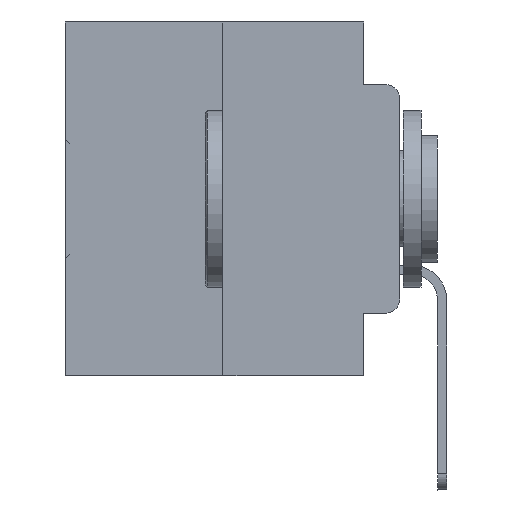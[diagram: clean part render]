
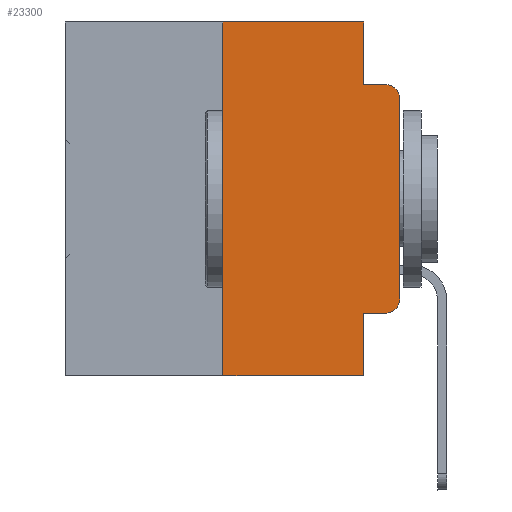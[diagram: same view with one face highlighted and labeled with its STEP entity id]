
A CAD part, left-side view. The second image highlights one B-rep face of the part: STEP entity #23300.
In plain terms, the highlighted planar face has unit normal (-1, 0, 0).
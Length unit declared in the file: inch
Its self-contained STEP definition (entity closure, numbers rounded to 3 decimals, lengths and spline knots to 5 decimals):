
#1575 = VERTEX_POINT ( 'NONE', #24179 ) ;
#1589 = EDGE_CURVE ( 'NONE', #19500, #1575, #29498, .T. ) ;
#2056 = CARTESIAN_POINT ( 'NONE',  ( 0., 0.473, 0. ) ) ;
#2067 = DIRECTION ( 'NONE',  ( 0., 0., 1. ) ) ;
#2554 = LINE ( 'NONE', #5208, #8796 ) ;
#2661 = CIRCLE ( 'NONE', #12740, 0.02 ) ;
#3149 = EDGE_CURVE ( 'NONE', #9847, #30426, #2661, .T. ) ;
#3550 = CARTESIAN_POINT ( 'NONE',  ( 0., 0.051, 0. ) ) ;
#4041 = CIRCLE ( 'NONE', #31563, 0.02 ) ;
#4110 = DIRECTION ( 'NONE',  ( 0., -1., 0. ) ) ;
#5208 = CARTESIAN_POINT ( 'NONE',  ( 0., 0.25, 0. ) ) ;
#5660 = CARTESIAN_POINT ( 'NONE',  ( 0., 0.051, -0.5 ) ) ;
#6188 = LINE ( 'NONE', #3550, #12052 ) ;
#7272 = VECTOR ( 'NONE', #7425, 39.37008 ) ;
#7425 = DIRECTION ( 'NONE',  ( 0., -1., 0. ) ) ;
#8256 = VECTOR ( 'NONE', #15714, 39.37008 ) ;
#8270 = CARTESIAN_POINT ( 'NONE',  ( 0., 0., -0.1085 ) ) ;
#8457 = DIRECTION ( 'NONE',  ( -1., 0., 0. ) ) ;
#8608 = CARTESIAN_POINT ( 'NONE',  ( 0., 0., 0. ) ) ;
#8796 = VECTOR ( 'NONE', #2067, 39.37008 ) ;
#9204 = VECTOR ( 'NONE', #17052, 39.37008 ) ;
#9364 = DIRECTION ( 'NONE',  ( 0., -1., 0. ) ) ;
#9847 = VERTEX_POINT ( 'NONE', #8270 ) ;
#9856 = DIRECTION ( 'NONE',  ( 1., 0., 0. ) ) ;
#11667 = ORIENTED_EDGE ( 'NONE', *, *, #15619, .T. ) ;
#12052 = VECTOR ( 'NONE', #23756, 39.37008 ) ;
#12657 = ORIENTED_EDGE ( 'NONE', *, *, #1589, .F. ) ;
#12740 = AXIS2_PLACEMENT_3D ( 'NONE', #23371, #8457, #28504 ) ;
#12898 = ORIENTED_EDGE ( 'NONE', *, *, #14330, .T. ) ;
#12933 = CARTESIAN_POINT ( 'NONE',  ( 0., 0.051, -0.0885 ) ) ;
#12967 = ORIENTED_EDGE ( 'NONE', *, *, #15094, .T. ) ;
#13583 = VECTOR ( 'NONE', #9364, 39.37008 ) ;
#13916 = CARTESIAN_POINT ( 'NONE',  ( 0., 0.473, 0. ) ) ;
#14045 = LINE ( 'NONE', #29971, #20692 ) ;
#14330 = EDGE_CURVE ( 'NONE', #26583, #25489, #25069, .T. ) ;
#14343 = CARTESIAN_POINT ( 'NONE',  ( 0., 0.02, -0.3915 ) ) ;
#15094 = EDGE_CURVE ( 'NONE', #24142, #9847, #18867, .T. ) ;
#15204 = CARTESIAN_POINT ( 'NONE',  ( 0., 0.473, -0.5 ) ) ;
#15619 = EDGE_CURVE ( 'NONE', #25489, #24142, #4041, .T. ) ;
#15714 = DIRECTION ( 'NONE',  ( 0., 0., 1. ) ) ;
#15797 = EDGE_CURVE ( 'NONE', #23424, #19500, #2554, .T. ) ;
#15815 = ORIENTED_EDGE ( 'NONE', *, *, #17167, .F. ) ;
#16565 = EDGE_CURVE ( 'NONE', #23424, #17661, #27963, .T. ) ;
#17052 = DIRECTION ( 'NONE',  ( 0., -1., 0. ) ) ;
#17167 = EDGE_CURVE ( 'NONE', #26583, #17661, #6188, .T. ) ;
#17392 = CARTESIAN_POINT ( 'NONE',  ( 0., 0.051, 0. ) ) ;
#17404 = VECTOR ( 'NONE', #30179, 39.37008 ) ;
#17661 = VERTEX_POINT ( 'NONE', #5660 ) ;
#18423 = EDGE_CURVE ( 'NONE', #1575, #20953, #27991, .T. ) ;
#18867 = LINE ( 'NONE', #8608, #8256 ) ;
#18978 = DIRECTION ( 'NONE',  ( 0., 0., -1. ) ) ;
#19500 = VERTEX_POINT ( 'NONE', #21232 ) ;
#19636 = FACE_OUTER_BOUND ( 'NONE', #29523, .T. ) ;
#19955 = DIRECTION ( 'NONE',  ( 0., 0., -1. ) ) ;
#20692 = VECTOR ( 'NONE', #4110, 39.37008 ) ;
#20931 = CARTESIAN_POINT ( 'NONE',  ( 0., 0.25, -0.5 ) ) ;
#20953 = VERTEX_POINT ( 'NONE', #12933 ) ;
#21232 = CARTESIAN_POINT ( 'NONE',  ( 0., 0.25, 0. ) ) ;
#22429 = CARTESIAN_POINT ( 'NONE',  ( 0., 0.051, -0.4115 ) ) ;
#23300 = ADVANCED_FACE ( 'NONE', ( #19636 ), #32566, .F. ) ;
#23371 = CARTESIAN_POINT ( 'NONE',  ( 0., 0.02, -0.1085 ) ) ;
#23424 = VERTEX_POINT ( 'NONE', #20931 ) ;
#23756 = DIRECTION ( 'NONE',  ( 0., 0., -1. ) ) ;
#24027 = CARTESIAN_POINT ( 'NONE',  ( 0., 0.02, -0.0885 ) ) ;
#24142 = VERTEX_POINT ( 'NONE', #27947 ) ;
#24179 = CARTESIAN_POINT ( 'NONE',  ( 0., 0.051, 0. ) ) ;
#24285 = DIRECTION ( 'NONE',  ( -1., 0., 0. ) ) ;
#25069 = LINE ( 'NONE', #31913, #13583 ) ;
#25405 = ORIENTED_EDGE ( 'NONE', *, *, #16565, .T. ) ;
#25489 = VERTEX_POINT ( 'NONE', #26130 ) ;
#26130 = CARTESIAN_POINT ( 'NONE',  ( 0., 0.02, -0.4115 ) ) ;
#26583 = VERTEX_POINT ( 'NONE', #22429 ) ;
#27185 = ORIENTED_EDGE ( 'NONE', *, *, #18423, .F. ) ;
#27795 = AXIS2_PLACEMENT_3D ( 'NONE', #2056, #9856, #19955 ) ;
#27947 = CARTESIAN_POINT ( 'NONE',  ( 0., 0., -0.3915 ) ) ;
#27963 = LINE ( 'NONE', #15204, #7272 ) ;
#27991 = LINE ( 'NONE', #17392, #17404 ) ;
#28391 = ORIENTED_EDGE ( 'NONE', *, *, #32333, .F. ) ;
#28504 = DIRECTION ( 'NONE',  ( 0., 0., -1. ) ) ;
#29498 = LINE ( 'NONE', #13916, #9204 ) ;
#29523 = EDGE_LOOP ( 'NONE', ( #12967, #32690, #28391, #27185, #12657, #29755, #25405, #15815, #12898, #11667 ) ) ;
#29755 = ORIENTED_EDGE ( 'NONE', *, *, #15797, .F. ) ;
#29971 = CARTESIAN_POINT ( 'NONE',  ( 0., 0.051, -0.0885 ) ) ;
#30179 = DIRECTION ( 'NONE',  ( 0., 0., -1. ) ) ;
#30426 = VERTEX_POINT ( 'NONE', #24027 ) ;
#31563 = AXIS2_PLACEMENT_3D ( 'NONE', #14343, #24285, #18978 ) ;
#31913 = CARTESIAN_POINT ( 'NONE',  ( 0., 0.051, -0.4115 ) ) ;
#32333 = EDGE_CURVE ( 'NONE', #20953, #30426, #14045, .T. ) ;
#32566 = PLANE ( 'NONE',  #27795 ) ;
#32690 = ORIENTED_EDGE ( 'NONE', *, *, #3149, .T. ) ;
